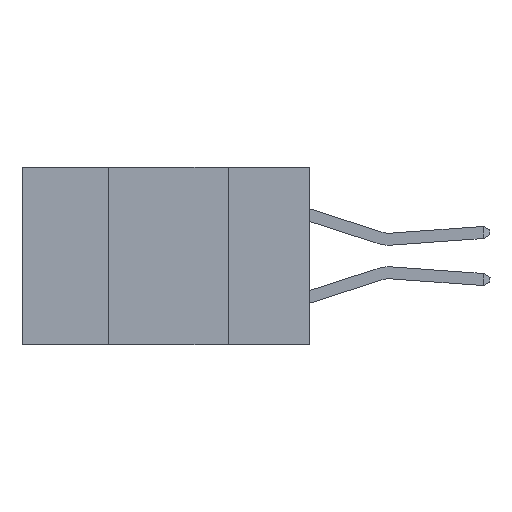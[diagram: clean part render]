
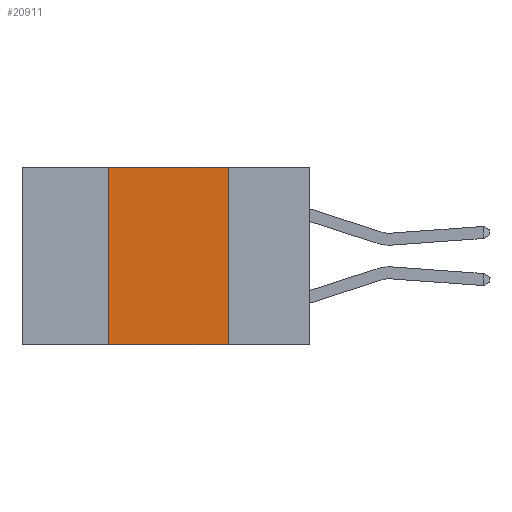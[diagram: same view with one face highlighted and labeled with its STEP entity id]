
A CAD part, left-side view. The second image highlights one B-rep face of the part: STEP entity #20911.
In plain terms, the highlighted planar face has unit normal (-1, 0, 0).
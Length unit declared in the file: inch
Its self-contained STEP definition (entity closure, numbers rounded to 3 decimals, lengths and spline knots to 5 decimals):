
#124 = CARTESIAN_POINT ( 'NONE',  ( 0., 0.42, 0. ) ) ;
#751 = LINE ( 'NONE', #1601, #4211 ) ;
#969 = CARTESIAN_POINT ( 'NONE',  ( 0., 0.17, 0. ) ) ;
#1157 = VERTEX_POINT ( 'NONE', #969 ) ;
#1601 = CARTESIAN_POINT ( 'NONE',  ( 0., 0.17, 0. ) ) ;
#1652 = CARTESIAN_POINT ( 'NONE',  ( 0., 0.17, -0.37 ) ) ;
#1748 = VERTEX_POINT ( 'NONE', #1652 ) ;
#1947 = DIRECTION ( 'NONE',  ( 0., -1., 0. ) ) ;
#2466 = AXIS2_PLACEMENT_3D ( 'NONE', #17722, #3018, #19384 ) ;
#2718 = LINE ( 'NONE', #124, #10772 ) ;
#3018 = DIRECTION ( 'NONE',  ( 1., 0., 0. ) ) ;
#4211 = VECTOR ( 'NONE', #16242, 39.37008 ) ;
#7073 = VERTEX_POINT ( 'NONE', #22681 ) ;
#7342 = EDGE_CURVE ( 'NONE', #1157, #1748, #751, .T. ) ;
#7793 = VECTOR ( 'NONE', #1947, 39.37008 ) ;
#8157 = EDGE_CURVE ( 'NONE', #7073, #1157, #20402, .T. ) ;
#8789 = EDGE_LOOP ( 'NONE', ( #11019, #13278, #23216, #9278 ) ) ;
#9278 = ORIENTED_EDGE ( 'NONE', *, *, #10657, .T. ) ;
#10657 = EDGE_CURVE ( 'NONE', #14638, #1748, #22605, .T. ) ;
#10772 = VECTOR ( 'NONE', #14756, 39.37008 ) ;
#11019 = ORIENTED_EDGE ( 'NONE', *, *, #7342, .F. ) ;
#12007 = PLANE ( 'NONE',  #2466 ) ;
#12990 = CARTESIAN_POINT ( 'NONE',  ( 0., 0.6, -0.37 ) ) ;
#13278 = ORIENTED_EDGE ( 'NONE', *, *, #8157, .F. ) ;
#13933 = DIRECTION ( 'NONE',  ( 0., -1., 0. ) ) ;
#14221 = FACE_OUTER_BOUND ( 'NONE', #8789, .T. ) ;
#14638 = VERTEX_POINT ( 'NONE', #22068 ) ;
#14756 = DIRECTION ( 'NONE',  ( 0., 0., 1. ) ) ;
#16242 = DIRECTION ( 'NONE',  ( 0., 0., -1. ) ) ;
#17722 = CARTESIAN_POINT ( 'NONE',  ( 0., 0.6, 0. ) ) ;
#19384 = DIRECTION ( 'NONE',  ( 0., 0., -1. ) ) ;
#20402 = LINE ( 'NONE', #21167, #20972 ) ;
#20911 = ADVANCED_FACE ( 'NONE', ( #14221 ), #12007, .F. ) ;
#20972 = VECTOR ( 'NONE', #13933, 39.37008 ) ;
#21167 = CARTESIAN_POINT ( 'NONE',  ( 0., 0.6, 0. ) ) ;
#21854 = EDGE_CURVE ( 'NONE', #14638, #7073, #2718, .T. ) ;
#22068 = CARTESIAN_POINT ( 'NONE',  ( 0., 0.42, -0.37 ) ) ;
#22605 = LINE ( 'NONE', #12990, #7793 ) ;
#22681 = CARTESIAN_POINT ( 'NONE',  ( 0., 0.42, 0. ) ) ;
#23216 = ORIENTED_EDGE ( 'NONE', *, *, #21854, .F. ) ;
